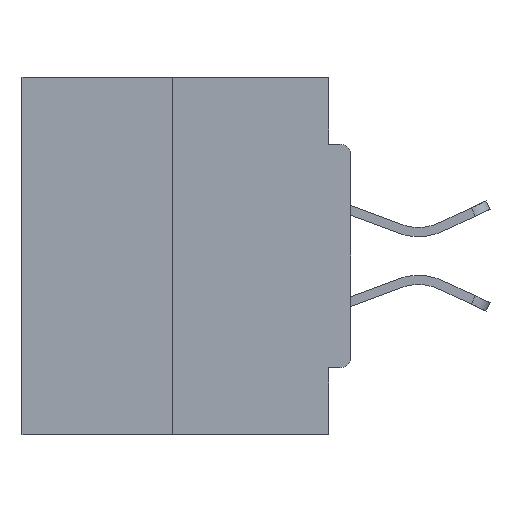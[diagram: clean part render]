
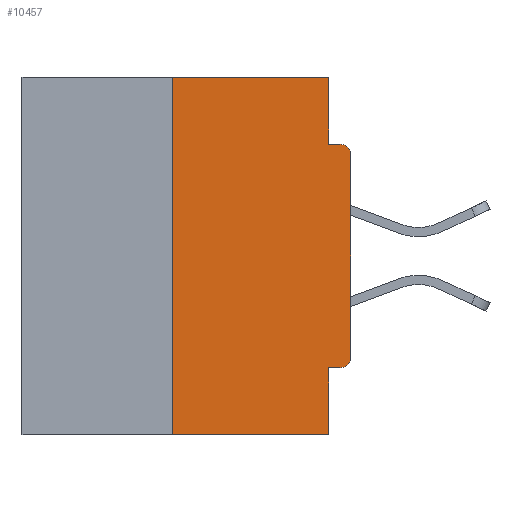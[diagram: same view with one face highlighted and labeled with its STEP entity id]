
A CAD part, left-side view. The second image highlights one B-rep face of the part: STEP entity #10457.
In plain terms, the highlighted planar face has unit normal (-1, 0, 0).
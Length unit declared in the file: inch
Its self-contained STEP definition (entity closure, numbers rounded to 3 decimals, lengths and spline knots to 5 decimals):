
#16 = CARTESIAN_POINT ( 'NONE',  ( 0., 0., -0.3915 ) ) ;
#174 = CARTESIAN_POINT ( 'NONE',  ( 0., 0.031, -0.4065 ) ) ;
#410 = EDGE_CURVE ( 'NONE', #10395, #23670, #33753, .T. ) ;
#665 = ORIENTED_EDGE ( 'NONE', *, *, #8740, .F. ) ;
#834 = EDGE_CURVE ( 'NONE', #13606, #27420, #27308, .T. ) ;
#1193 = DIRECTION ( 'NONE',  ( 0., -1., 0. ) ) ;
#1364 = VECTOR ( 'NONE', #24876, 39.37008 ) ;
#1528 = CARTESIAN_POINT ( 'NONE',  ( 0., 0.46, 0. ) ) ;
#2432 = VERTEX_POINT ( 'NONE', #38611 ) ;
#3491 = VECTOR ( 'NONE', #13715, 39.37008 ) ;
#5057 = CARTESIAN_POINT ( 'NONE',  ( 0., 0.25, 0. ) ) ;
#7127 = CARTESIAN_POINT ( 'NONE',  ( 0., 0., -0.0935 ) ) ;
#7264 = DIRECTION ( 'NONE',  ( 1., 0., 0. ) ) ;
#8740 = EDGE_CURVE ( 'NONE', #23670, #38898, #11884, .T. ) ;
#9183 = EDGE_LOOP ( 'NONE', ( #665, #36630, #31191, #35076, #13749, #40039, #35698, #23726, #35922, #26577 ) ) ;
#10346 = CARTESIAN_POINT ( 'NONE',  ( 0., 0.031, -0.5 ) ) ;
#10395 = VERTEX_POINT ( 'NONE', #32487 ) ;
#10457 = ADVANCED_FACE ( 'NONE', ( #28672 ), #20277, .F. ) ;
#10631 = DIRECTION ( 'NONE',  ( 0., 0., -1. ) ) ;
#11884 = LINE ( 'NONE', #1528, #3491 ) ;
#13308 = DIRECTION ( 'NONE',  ( 0., 0., -1. ) ) ;
#13606 = VERTEX_POINT ( 'NONE', #18675 ) ;
#13715 = DIRECTION ( 'NONE',  ( 0., -1., 0. ) ) ;
#13749 = ORIENTED_EDGE ( 'NONE', *, *, #33551, .F. ) ;
#13779 = CARTESIAN_POINT ( 'NONE',  ( 0., 0.015, -0.3915 ) ) ;
#14098 = CARTESIAN_POINT ( 'NONE',  ( 0., 0., 0. ) ) ;
#14598 = EDGE_CURVE ( 'NONE', #10395, #35139, #37964, .T. ) ;
#14600 = VECTOR ( 'NONE', #1193, 39.37008 ) ;
#14633 = EDGE_CURVE ( 'NONE', #18979, #15732, #36465, .T. ) ;
#15366 = VECTOR ( 'NONE', #10631, 39.37008 ) ;
#15732 = VERTEX_POINT ( 'NONE', #16 ) ;
#16359 = CARTESIAN_POINT ( 'NONE',  ( 0., 0.015, -0.1085 ) ) ;
#16749 = LINE ( 'NONE', #14098, #28777 ) ;
#16750 = DIRECTION ( 'NONE',  ( -1., 0., 0. ) ) ;
#16799 = CARTESIAN_POINT ( 'NONE',  ( 0., 0.46, -0.5 ) ) ;
#16857 = VECTOR ( 'NONE', #31320, 39.37008 ) ;
#17179 = CARTESIAN_POINT ( 'NONE',  ( 0., 0.031, -0.5 ) ) ;
#17671 = LINE ( 'NONE', #20562, #1364 ) ;
#18675 = CARTESIAN_POINT ( 'NONE',  ( 0., 0.031, -0.0935 ) ) ;
#18883 = VECTOR ( 'NONE', #25587, 39.37008 ) ;
#18979 = VERTEX_POINT ( 'NONE', #27149 ) ;
#18988 = EDGE_CURVE ( 'NONE', #15732, #2432, #16749, .T. ) ;
#19165 = AXIS2_PLACEMENT_3D ( 'NONE', #26229, #7264, #23495 ) ;
#20030 = DIRECTION ( 'NONE',  ( 0., 0., -1. ) ) ;
#20141 = CIRCLE ( 'NONE', #39876, 0.015 ) ;
#20277 = PLANE ( 'NONE',  #19165 ) ;
#20562 = CARTESIAN_POINT ( 'NONE',  ( 0., 0., -0.4065 ) ) ;
#20966 = DIRECTION ( 'NONE',  ( 0., 0., -1. ) ) ;
#21905 = CARTESIAN_POINT ( 'NONE',  ( 0., 0.015, -0.0935 ) ) ;
#22863 = LINE ( 'NONE', #29040, #15366 ) ;
#23495 = DIRECTION ( 'NONE',  ( 0., 0., -1. ) ) ;
#23670 = VERTEX_POINT ( 'NONE', #5057 ) ;
#23726 = ORIENTED_EDGE ( 'NONE', *, *, #31555, .T. ) ;
#24857 = VERTEX_POINT ( 'NONE', #174 ) ;
#24876 = DIRECTION ( 'NONE',  ( 0., 1., 0. ) ) ;
#25587 = DIRECTION ( 'NONE',  ( 0., -1., 0. ) ) ;
#25955 = EDGE_CURVE ( 'NONE', #38898, #13606, #22863, .T. ) ;
#26229 = CARTESIAN_POINT ( 'NONE',  ( 0., 0.46, 0. ) ) ;
#26542 = EDGE_CURVE ( 'NONE', #24857, #35139, #27717, .T. ) ;
#26544 = AXIS2_PLACEMENT_3D ( 'NONE', #13779, #29575, #20030 ) ;
#26577 = ORIENTED_EDGE ( 'NONE', *, *, #25955, .F. ) ;
#27149 = CARTESIAN_POINT ( 'NONE',  ( 0., 0.015, -0.4065 ) ) ;
#27199 = VECTOR ( 'NONE', #20966, 39.37008 ) ;
#27308 = LINE ( 'NONE', #7127, #18883 ) ;
#27420 = VERTEX_POINT ( 'NONE', #21905 ) ;
#27717 = LINE ( 'NONE', #17179, #27199 ) ;
#28266 = CARTESIAN_POINT ( 'NONE',  ( 0., 0.25, 0. ) ) ;
#28672 = FACE_OUTER_BOUND ( 'NONE', #9183, .T. ) ;
#28777 = VECTOR ( 'NONE', #33108, 39.37008 ) ;
#29040 = CARTESIAN_POINT ( 'NONE',  ( 0., 0.031, 0. ) ) ;
#29575 = DIRECTION ( 'NONE',  ( -1., 0., 0. ) ) ;
#31191 = ORIENTED_EDGE ( 'NONE', *, *, #14598, .T. ) ;
#31320 = DIRECTION ( 'NONE',  ( 0., 0., 1. ) ) ;
#31555 = EDGE_CURVE ( 'NONE', #2432, #27420, #20141, .T. ) ;
#32487 = CARTESIAN_POINT ( 'NONE',  ( 0., 0.25, -0.5 ) ) ;
#33108 = DIRECTION ( 'NONE',  ( 0., 0., 1. ) ) ;
#33551 = EDGE_CURVE ( 'NONE', #18979, #24857, #17671, .T. ) ;
#33753 = LINE ( 'NONE', #28266, #16857 ) ;
#34500 = CARTESIAN_POINT ( 'NONE',  ( 0., 0.031, 0. ) ) ;
#35076 = ORIENTED_EDGE ( 'NONE', *, *, #26542, .F. ) ;
#35139 = VERTEX_POINT ( 'NONE', #10346 ) ;
#35698 = ORIENTED_EDGE ( 'NONE', *, *, #18988, .T. ) ;
#35922 = ORIENTED_EDGE ( 'NONE', *, *, #834, .F. ) ;
#36465 = CIRCLE ( 'NONE', #26544, 0.015 ) ;
#36630 = ORIENTED_EDGE ( 'NONE', *, *, #410, .F. ) ;
#37964 = LINE ( 'NONE', #16799, #14600 ) ;
#38611 = CARTESIAN_POINT ( 'NONE',  ( 0., 0., -0.1085 ) ) ;
#38898 = VERTEX_POINT ( 'NONE', #34500 ) ;
#39876 = AXIS2_PLACEMENT_3D ( 'NONE', #16359, #16750, #13308 ) ;
#40039 = ORIENTED_EDGE ( 'NONE', *, *, #14633, .T. ) ;
